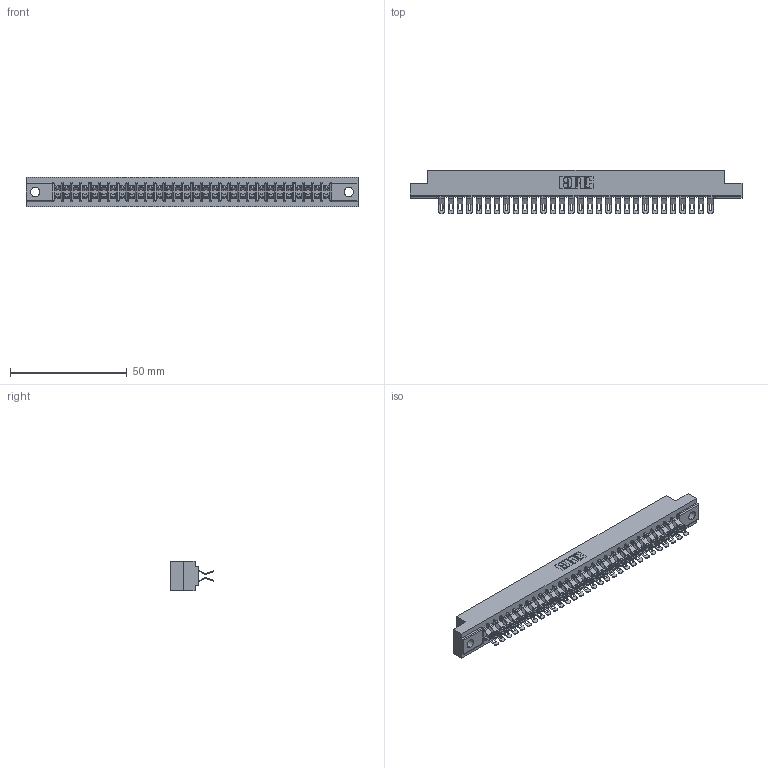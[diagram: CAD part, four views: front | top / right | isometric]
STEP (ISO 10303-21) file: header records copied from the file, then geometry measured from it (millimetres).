
FILE_DESCRIPTION (( 'STEP AP203' ), '1' );
FILE_NAME ('307-060-555-204.STEP', '2019-09-06T15:32:12', ( '' ), ( '' ), 'SwSTEP 2.0', 'SolidWorks 2016', '' );
FILE_SCHEMA (( 'CONFIG_CONTROL_DESIGN' ));
Length unit declared in the file: inch
Products named in the file (3): 307-060-555-204; 307-290-001_555; 307 Part_.156 Dia Mounting Holes
Assembly tree (61 placements, depth 2):
  307-060-555-204
    307 Part_.156 Dia Mounting Holes
    307-290-001_555  x60
Bounding box: 141.88 x 18.75 x 12.7 mm (x, y, z)
Volume: 15075.5 mm3; surface area: 19029.2 mm2
Topology: 61 solids, 61 shells, 3823 faces, 11219 edges, 7314 vertices
Faces by surface type: plane 2124, cylinder 1637, sphere 62
Entity records: 29113 total; most frequent: CARTESIAN_POINT 4776, ORIENTED_EDGE 4732, DIRECTION 4682, EDGE_CURVE 2366, VECTOR 1806, LINE 1806, VERTEX_POINT 1532, AXIS2_PLACEMENT_3D 1438
